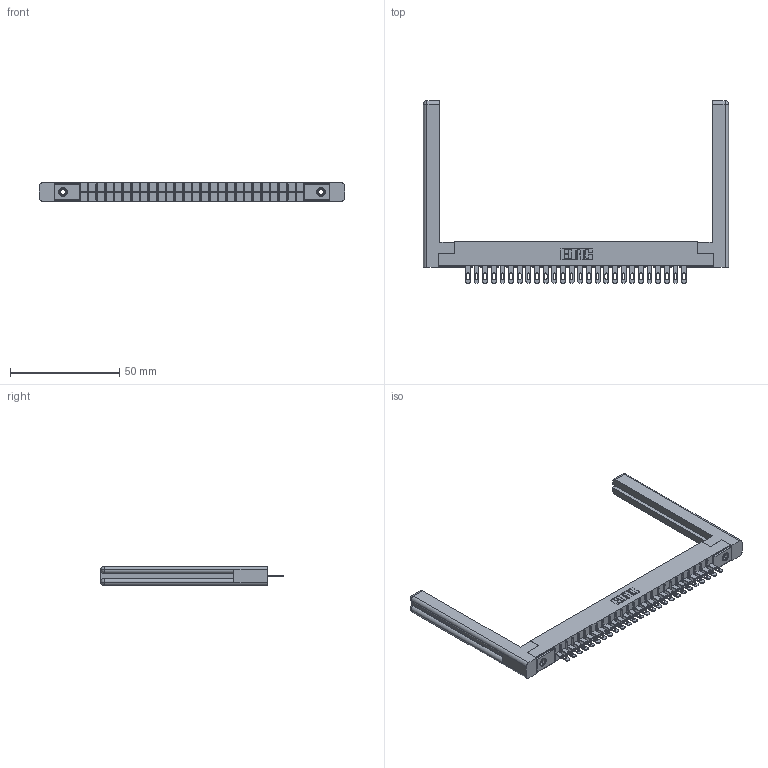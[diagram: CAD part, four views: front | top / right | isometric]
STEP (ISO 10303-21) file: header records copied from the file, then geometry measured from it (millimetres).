
FILE_DESCRIPTION (( 'STEP AP203' ), '1' );
FILE_NAME ('306-026-400-158.STEP', '2020-09-21T23:06:02', ( '' ), ( '' ), 'SwSTEP 2.0', 'SolidWorks 2020', '' );
FILE_SCHEMA (( 'CONFIG_CONTROL_DESIGN' ));
Length unit declared in the file: inch
Products named in the file (5): 345-250-001_345-250-001-102; 307-220-058; 306-026-400-158; 306 Part_.156 Dia; 306-290-001_100
Assembly tree (31 placements, depth 2):
  306-026-400-158
    306 Part_.156 Dia
    306-290-001_100  x26
    345-250-001_345-250-001-102  x2
    307-220-058  x2
Bounding box: 139.65 x 83.52 x 8.71 mm (x, y, z)
Volume: 17294.2 mm3; surface area: 20104.7 mm2
Topology: 31 solids, 31 shells, 2234 faces, 6260 edges, 4020 vertices
Faces by surface type: plane 1452, cylinder 654, sphere 104, cone 12, torus 12
Entity records: 29116 total; most frequent: CARTESIAN_POINT 4896, ORIENTED_EDGE 4794, DIRECTION 4785, EDGE_CURVE 2397, VECTOR 1859, LINE 1859, VERTEX_POINT 1520, AXIS2_PLACEMENT_3D 1463
